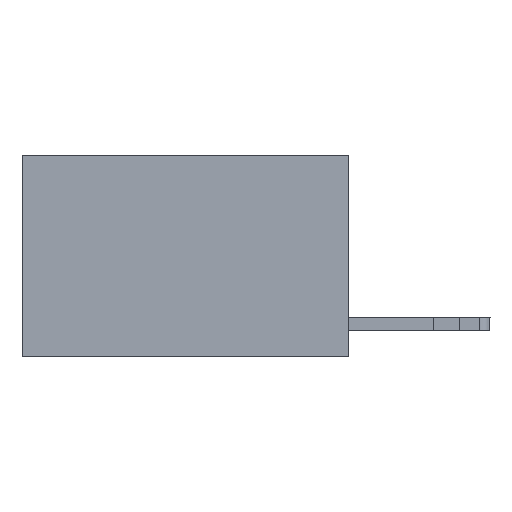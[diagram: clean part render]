
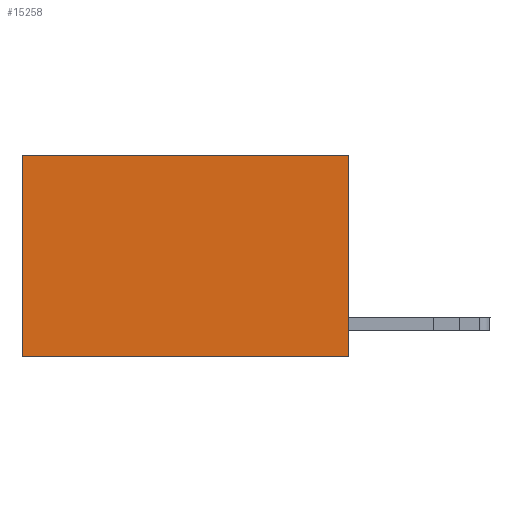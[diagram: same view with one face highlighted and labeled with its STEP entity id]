
A CAD part, left-side view. The second image highlights one B-rep face of the part: STEP entity #15258.
In plain terms, the highlighted planar face has unit normal (-1, 0, 0).
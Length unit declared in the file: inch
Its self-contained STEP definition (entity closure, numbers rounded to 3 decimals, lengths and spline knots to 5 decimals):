
#598 = DIRECTION ( 'NONE',  ( 0., 1., 0. ) ) ;
#946 = VERTEX_POINT ( 'NONE', #12331 ) ;
#1120 = DIRECTION ( 'NONE',  ( 0., 0., -1. ) ) ;
#1762 = EDGE_LOOP ( 'NONE', ( #10147, #23261, #19803, #11905 ) ) ;
#2172 = EDGE_CURVE ( 'NONE', #2701, #946, #26671, .T. ) ;
#2611 = DIRECTION ( 'NONE',  ( 0., 0., -1. ) ) ;
#2701 = VERTEX_POINT ( 'NONE', #4126 ) ;
#3331 = CARTESIAN_POINT ( 'NONE',  ( 0.2625, 0., 0. ) ) ;
#3730 = DIRECTION ( 'NONE',  ( 0., 1., 0. ) ) ;
#4126 = CARTESIAN_POINT ( 'NONE',  ( 0.2625, 0., -0.37 ) ) ;
#4499 = DIRECTION ( 'NONE',  ( 0., 0., -1. ) ) ;
#4502 = EDGE_CURVE ( 'NONE', #20225, #946, #28109, .T. ) ;
#4637 = CARTESIAN_POINT ( 'NONE',  ( 0.2625, 0.6, 0. ) ) ;
#5568 = CARTESIAN_POINT ( 'NONE',  ( 0.2625, 0., 0. ) ) ;
#5752 = VECTOR ( 'NONE', #4499, 39.37008 ) ;
#7356 = VERTEX_POINT ( 'NONE', #3331 ) ;
#7715 = CARTESIAN_POINT ( 'NONE',  ( 0.2625, 0., 0. ) ) ;
#9519 = AXIS2_PLACEMENT_3D ( 'NONE', #5568, #18065, #1120 ) ;
#9982 = LINE ( 'NONE', #7715, #20705 ) ;
#10147 = ORIENTED_EDGE ( 'NONE', *, *, #4502, .T. ) ;
#11572 = CARTESIAN_POINT ( 'NONE',  ( 0.2625, 0., -0.37 ) ) ;
#11905 = ORIENTED_EDGE ( 'NONE', *, *, #25350, .T. ) ;
#12331 = CARTESIAN_POINT ( 'NONE',  ( 0.2625, 0.6, -0.37 ) ) ;
#15258 = ADVANCED_FACE ( 'NONE', ( #20348 ), #25071, .F. ) ;
#15592 = LINE ( 'NONE', #26148, #5752 ) ;
#15679 = VECTOR ( 'NONE', #598, 39.37008 ) ;
#16383 = VECTOR ( 'NONE', #2611, 39.37008 ) ;
#18065 = DIRECTION ( 'NONE',  ( 1., 0., 0. ) ) ;
#19803 = ORIENTED_EDGE ( 'NONE', *, *, #25934, .F. ) ;
#20225 = VERTEX_POINT ( 'NONE', #24797 ) ;
#20348 = FACE_OUTER_BOUND ( 'NONE', #1762, .T. ) ;
#20705 = VECTOR ( 'NONE', #3730, 39.37008 ) ;
#23261 = ORIENTED_EDGE ( 'NONE', *, *, #2172, .F. ) ;
#24797 = CARTESIAN_POINT ( 'NONE',  ( 0.2625, 0.6, 0. ) ) ;
#25071 = PLANE ( 'NONE',  #9519 ) ;
#25350 = EDGE_CURVE ( 'NONE', #7356, #20225, #9982, .T. ) ;
#25934 = EDGE_CURVE ( 'NONE', #7356, #2701, #15592, .T. ) ;
#26148 = CARTESIAN_POINT ( 'NONE',  ( 0.2625, 0., 0. ) ) ;
#26671 = LINE ( 'NONE', #11572, #15679 ) ;
#28109 = LINE ( 'NONE', #4637, #16383 ) ;
